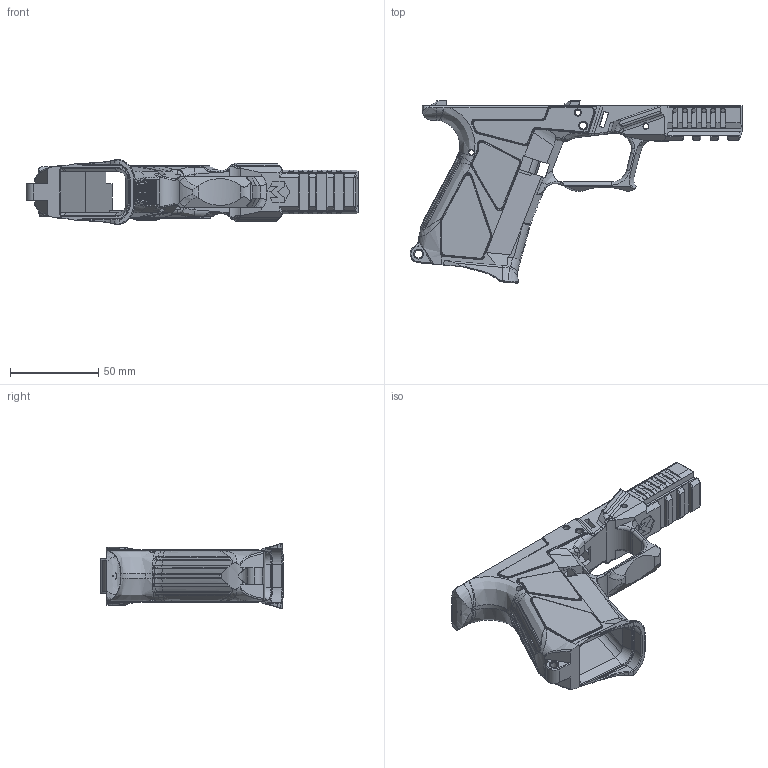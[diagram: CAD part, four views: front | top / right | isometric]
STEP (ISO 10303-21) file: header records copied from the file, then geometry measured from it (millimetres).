
FILE_DESCRIPTION (( 'STEP AP214' ), '1' );
FILE_NAME ('Schnitzel G19 Frame v1-5 STEP.STEP', '2022-10-09T22:27:22', ( '' ), ( '' ), 'SwSTEP 2.0', 'SolidWorks 2020', '' );
FILE_SCHEMA (( 'AUTOMOTIVE_DESIGN' ));
Length unit declared in the file: inch
Products named in the file (1): Schnitzel G19 Frame v1-5 STEP
Bounding box: 187.65 x 103.2 x 36.58 mm (x, y, z)
Volume: 92478.2 mm3; surface area: 48710 mm2
Topology: 1 solids, 4 shells, 1735 faces, 4616 edges, 2900 vertices
Faces by surface type: plane 730, cylinder 422, bspline 410, cone 83, torus 70, sphere 20
Entity records: 83258 total; most frequent: CARTESIAN_POINT 43758, ORIENTED_EDGE 9232, DIRECTION 6707, EDGE_CURVE 4616, VERTEX_POINT 2900, LINE 2407, VECTOR 2407, AXIS2_PLACEMENT_3D 2150
